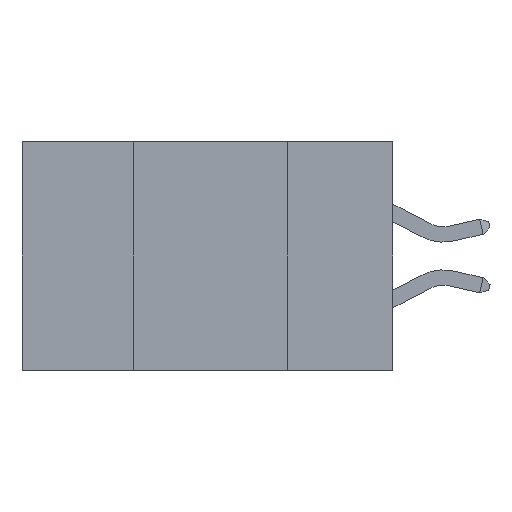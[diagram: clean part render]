
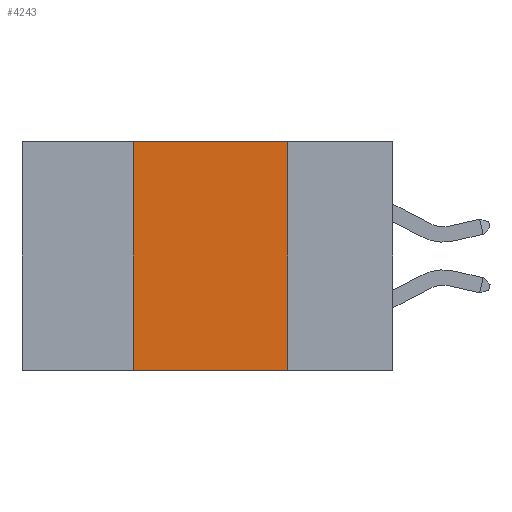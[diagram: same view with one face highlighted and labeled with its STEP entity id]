
A CAD part, left-side view. The second image highlights one B-rep face of the part: STEP entity #4243.
In plain terms, the highlighted planar face has unit normal (-1, 0, 0).
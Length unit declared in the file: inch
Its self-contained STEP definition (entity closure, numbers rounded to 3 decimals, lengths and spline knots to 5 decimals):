
#159 = DIRECTION ( 'NONE',  ( 0., 0., 1. ) ) ;
#526 = CARTESIAN_POINT ( 'NONE',  ( 0., 0.42, 0. ) ) ;
#547 = VERTEX_POINT ( 'NONE', #12836 ) ;
#582 = AXIS2_PLACEMENT_3D ( 'NONE', #6519, #10786, #4068 ) ;
#1294 = DIRECTION ( 'NONE',  ( 0., -1., 0. ) ) ;
#1685 = EDGE_CURVE ( 'NONE', #8268, #547, #6455, .T. ) ;
#1726 = VECTOR ( 'NONE', #1294, 39.37008 ) ;
#2144 = ORIENTED_EDGE ( 'NONE', *, *, #5307, .F. ) ;
#3011 = CARTESIAN_POINT ( 'NONE',  ( 0., 0.17, 0. ) ) ;
#4068 = DIRECTION ( 'NONE',  ( 0., 0., -1. ) ) ;
#4243 = ADVANCED_FACE ( 'NONE', ( #10964 ), #6469, .F. ) ;
#5307 = EDGE_CURVE ( 'NONE', #8268, #8225, #8080, .T. ) ;
#5693 = EDGE_LOOP ( 'NONE', ( #12754, #6837, #2144, #10051 ) ) ;
#6217 = VECTOR ( 'NONE', #11463, 39.37008 ) ;
#6455 = LINE ( 'NONE', #13689, #12935 ) ;
#6469 = PLANE ( 'NONE',  #582 ) ;
#6506 = EDGE_CURVE ( 'NONE', #7015, #547, #13030, .T. ) ;
#6519 = CARTESIAN_POINT ( 'NONE',  ( 0., 0.6, 0. ) ) ;
#6837 = ORIENTED_EDGE ( 'NONE', *, *, #10625, .F. ) ;
#7015 = VERTEX_POINT ( 'NONE', #3011 ) ;
#8013 = CARTESIAN_POINT ( 'NONE',  ( 0., 0.6, 0. ) ) ;
#8080 = LINE ( 'NONE', #13305, #14383 ) ;
#8225 = VERTEX_POINT ( 'NONE', #526 ) ;
#8268 = VERTEX_POINT ( 'NONE', #8417 ) ;
#8417 = CARTESIAN_POINT ( 'NONE',  ( 0., 0.42, -0.37 ) ) ;
#9124 = DIRECTION ( 'NONE',  ( 0., -1., 0. ) ) ;
#9949 = LINE ( 'NONE', #8013, #1726 ) ;
#10051 = ORIENTED_EDGE ( 'NONE', *, *, #1685, .T. ) ;
#10625 = EDGE_CURVE ( 'NONE', #8225, #7015, #9949, .T. ) ;
#10786 = DIRECTION ( 'NONE',  ( 1., 0., 0. ) ) ;
#10964 = FACE_OUTER_BOUND ( 'NONE', #5693, .T. ) ;
#11463 = DIRECTION ( 'NONE',  ( 0., 0., -1. ) ) ;
#12754 = ORIENTED_EDGE ( 'NONE', *, *, #6506, .F. ) ;
#12836 = CARTESIAN_POINT ( 'NONE',  ( 0., 0.17, -0.37 ) ) ;
#12935 = VECTOR ( 'NONE', #9124, 39.37008 ) ;
#13030 = LINE ( 'NONE', #13629, #6217 ) ;
#13305 = CARTESIAN_POINT ( 'NONE',  ( 0., 0.42, 0. ) ) ;
#13629 = CARTESIAN_POINT ( 'NONE',  ( 0., 0.17, 0. ) ) ;
#13689 = CARTESIAN_POINT ( 'NONE',  ( 0., 0.6, -0.37 ) ) ;
#14383 = VECTOR ( 'NONE', #159, 39.37008 ) ;
